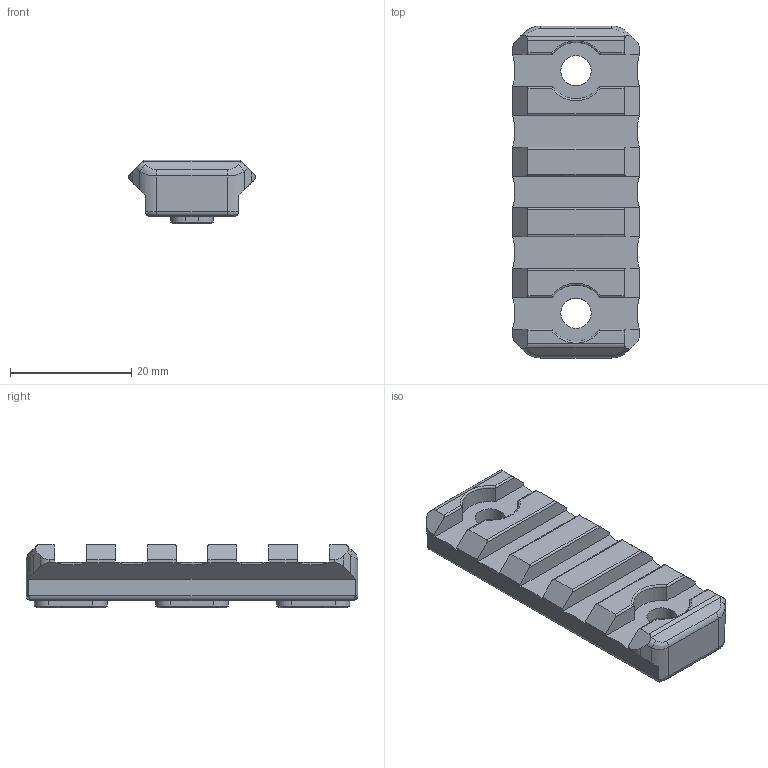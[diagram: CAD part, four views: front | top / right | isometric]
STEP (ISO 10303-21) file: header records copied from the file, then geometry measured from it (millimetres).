
FILE_DESCRIPTION(/* description */ (''),/* implementation_level */ '2;1');
FILE_NAME(/* name */ 'MLok - Picatinny Adaptor Rail.step',/* time_stamp */ '2021-06-03T17:14:39-04:00',/* author */ (''),/* organization */ (''),/* preprocessor_version */ 'ST-DEVELOPER v18.1',/* originating_system */ 'Autodesk Translation Framework v10.9.0.1377',/* authorisation */ '');
FILE_SCHEMA (('AUTOMOTIVE_DESIGN { 1 0 10303 214 3 1 1 }'));
Length unit declared in the file: millimetre
Products named in the file (1): MLok - Picatinny Adaptor Rail
Bounding box: 20.91 x 54.75 x 10.52 mm (x, y, z)
Volume: 7068.6 mm3; surface area: 3866.1 mm2
Topology: 1 solids, 1 shells, 187 faces, 468 edges, 286 vertices
Faces by surface type: plane 93, cylinder 62, cone 18, torus 10, bspline 4
Full cylindrical faces by diameter (mm): 5 x2
Entity records: 5738 total; most frequent: CARTESIAN_POINT 1174, DIRECTION 968, ORIENTED_EDGE 936, EDGE_CURVE 468, AXIS2_PLACEMENT_3D 336, LINE 296, VECTOR 296, VERTEX_POINT 286
